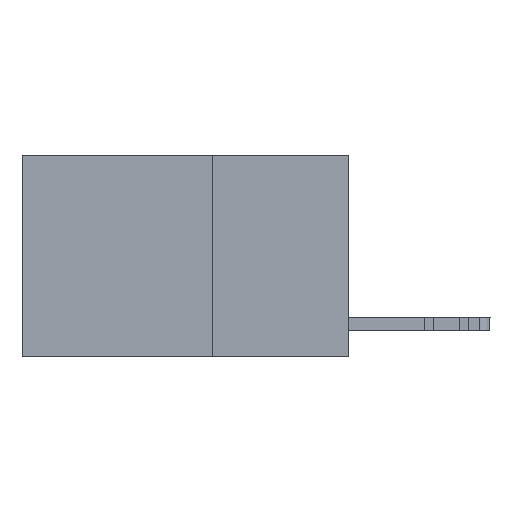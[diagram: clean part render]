
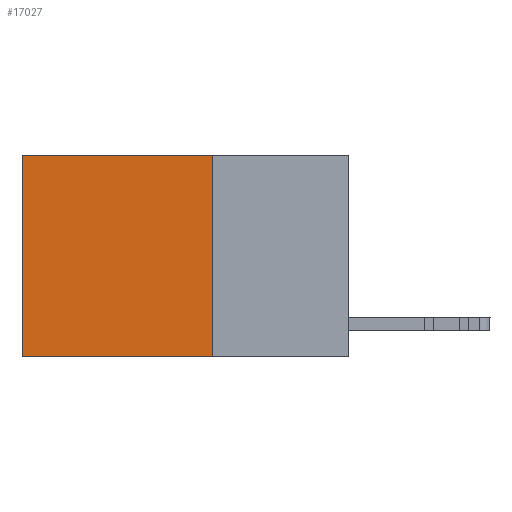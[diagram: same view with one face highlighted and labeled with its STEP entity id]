
A CAD part, left-side view. The second image highlights one B-rep face of the part: STEP entity #17027.
In plain terms, the highlighted planar face has unit normal (-1, 0, 0).
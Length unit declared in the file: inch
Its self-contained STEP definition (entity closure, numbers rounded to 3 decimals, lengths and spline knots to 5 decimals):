
#1126 = ORIENTED_EDGE ( 'NONE', *, *, #26500, .F. ) ;
#1659 = DIRECTION ( 'NONE',  ( 0., 1., 0. ) ) ;
#2226 = VECTOR ( 'NONE', #25532, 39.37008 ) ;
#2548 = FACE_OUTER_BOUND ( 'NONE', #3197, .T. ) ;
#3197 = EDGE_LOOP ( 'NONE', ( #25888, #24249, #1126, #15978 ) ) ;
#4290 = LINE ( 'NONE', #18092, #16017 ) ;
#6345 = VERTEX_POINT ( 'NONE', #28592 ) ;
#6925 = VECTOR ( 'NONE', #1659, 39.37008 ) ;
#7603 = CARTESIAN_POINT ( 'NONE',  ( 0.2625, 0.6, 0. ) ) ;
#7978 = VERTEX_POINT ( 'NONE', #11285 ) ;
#8603 = LINE ( 'NONE', #9500, #2226 ) ;
#8796 = CARTESIAN_POINT ( 'NONE',  ( 0.2625, 0.25, 0. ) ) ;
#9500 = CARTESIAN_POINT ( 'NONE',  ( 0.2625, 0.25, -0.37 ) ) ;
#9968 = DIRECTION ( 'NONE',  ( 0., 0., -1. ) ) ;
#11285 = CARTESIAN_POINT ( 'NONE',  ( 0.2625, 0.6, -0.37 ) ) ;
#11609 = CARTESIAN_POINT ( 'NONE',  ( 0.2625, 0.25, 0. ) ) ;
#11667 = DIRECTION ( 'NONE',  ( 0., 0., -1. ) ) ;
#12101 = VERTEX_POINT ( 'NONE', #11609 ) ;
#15978 = ORIENTED_EDGE ( 'NONE', *, *, #17996, .T. ) ;
#16017 = VECTOR ( 'NONE', #20377, 39.37008 ) ;
#17027 = ADVANCED_FACE ( 'NONE', ( #2548 ), #25297, .F. ) ;
#17165 = EDGE_CURVE ( 'NONE', #20141, #7978, #17593, .T. ) ;
#17593 = LINE ( 'NONE', #7603, #22922 ) ;
#17996 = EDGE_CURVE ( 'NONE', #12101, #20141, #19245, .T. ) ;
#18092 = CARTESIAN_POINT ( 'NONE',  ( 0.2625, 0.25, 0. ) ) ;
#18511 = CARTESIAN_POINT ( 'NONE',  ( 0.2625, 0.25, 0. ) ) ;
#18591 = AXIS2_PLACEMENT_3D ( 'NONE', #18511, #25396, #11667 ) ;
#19245 = LINE ( 'NONE', #8796, #6925 ) ;
#20141 = VERTEX_POINT ( 'NONE', #25631 ) ;
#20377 = DIRECTION ( 'NONE',  ( 0., 0., -1. ) ) ;
#22922 = VECTOR ( 'NONE', #9968, 39.37008 ) ;
#24249 = ORIENTED_EDGE ( 'NONE', *, *, #28921, .F. ) ;
#25297 = PLANE ( 'NONE',  #18591 ) ;
#25396 = DIRECTION ( 'NONE',  ( 1., 0., 0. ) ) ;
#25532 = DIRECTION ( 'NONE',  ( 0., 1., 0. ) ) ;
#25631 = CARTESIAN_POINT ( 'NONE',  ( 0.2625, 0.6, 0. ) ) ;
#25888 = ORIENTED_EDGE ( 'NONE', *, *, #17165, .T. ) ;
#26500 = EDGE_CURVE ( 'NONE', #12101, #6345, #4290, .T. ) ;
#28592 = CARTESIAN_POINT ( 'NONE',  ( 0.2625, 0.25, -0.37 ) ) ;
#28921 = EDGE_CURVE ( 'NONE', #6345, #7978, #8603, .T. ) ;
